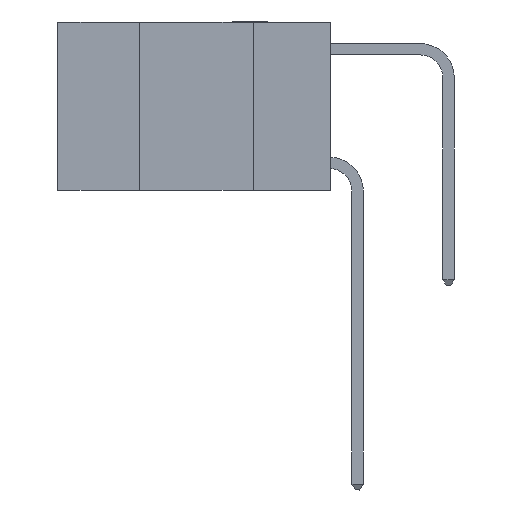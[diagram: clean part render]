
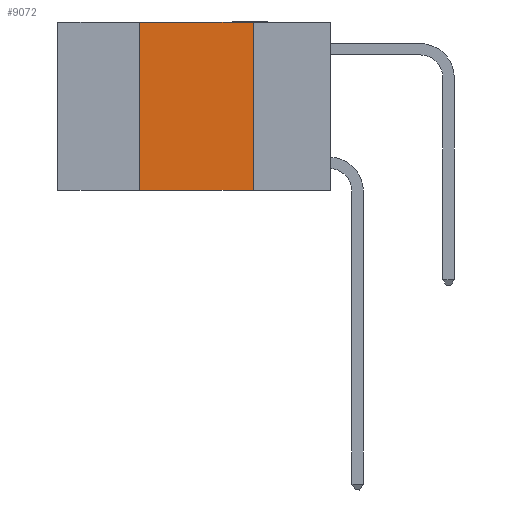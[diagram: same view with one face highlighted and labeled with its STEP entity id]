
A CAD part, left-side view. The second image highlights one B-rep face of the part: STEP entity #9072.
In plain terms, the highlighted planar face has unit normal (-1, 0, 0).
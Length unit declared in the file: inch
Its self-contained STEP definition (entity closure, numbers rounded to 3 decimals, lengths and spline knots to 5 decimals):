
#409 = CARTESIAN_POINT ( 'NONE',  ( 0., 0.42, 0. ) ) ;
#1998 = ORIENTED_EDGE ( 'NONE', *, *, #14082, .F. ) ;
#2023 = DIRECTION ( 'NONE',  ( 0., -1., 0. ) ) ;
#2148 = PLANE ( 'NONE',  #6805 ) ;
#3165 = ORIENTED_EDGE ( 'NONE', *, *, #5633, .F. ) ;
#3725 = LINE ( 'NONE', #13849, #8418 ) ;
#4829 = CARTESIAN_POINT ( 'NONE',  ( 0., 0.42, -0.37 ) ) ;
#5521 = VERTEX_POINT ( 'NONE', #15362 ) ;
#5633 = EDGE_CURVE ( 'NONE', #11752, #13836, #15517, .T. ) ;
#5691 = EDGE_LOOP ( 'NONE', ( #15381, #1998, #3165, #9033 ) ) ;
#5733 = EDGE_CURVE ( 'NONE', #11752, #10014, #7195, .T. ) ;
#5978 = DIRECTION ( 'NONE',  ( 0., 0., -1. ) ) ;
#6142 = DIRECTION ( 'NONE',  ( 0., 0., -1. ) ) ;
#6805 = AXIS2_PLACEMENT_3D ( 'NONE', #7239, #12229, #5978 ) ;
#7195 = LINE ( 'NONE', #13567, #16121 ) ;
#7239 = CARTESIAN_POINT ( 'NONE',  ( 0., 0.6, 0. ) ) ;
#8418 = VECTOR ( 'NONE', #6142, 39.37008 ) ;
#8916 = LINE ( 'NONE', #13835, #11642 ) ;
#9033 = ORIENTED_EDGE ( 'NONE', *, *, #5733, .T. ) ;
#9072 = ADVANCED_FACE ( 'NONE', ( #10893 ), #2148, .F. ) ;
#9412 = CARTESIAN_POINT ( 'NONE',  ( 0., 0.42, 0. ) ) ;
#9589 = EDGE_CURVE ( 'NONE', #5521, #10014, #3725, .T. ) ;
#10014 = VERTEX_POINT ( 'NONE', #16158 ) ;
#10372 = DIRECTION ( 'NONE',  ( 0., 0., 1. ) ) ;
#10893 = FACE_OUTER_BOUND ( 'NONE', #5691, .T. ) ;
#11642 = VECTOR ( 'NONE', #12528, 39.37008 ) ;
#11752 = VERTEX_POINT ( 'NONE', #4829 ) ;
#12229 = DIRECTION ( 'NONE',  ( 1., 0., 0. ) ) ;
#12421 = VECTOR ( 'NONE', #10372, 39.37008 ) ;
#12528 = DIRECTION ( 'NONE',  ( 0., -1., 0. ) ) ;
#13567 = CARTESIAN_POINT ( 'NONE',  ( 0., 0.6, -0.37 ) ) ;
#13836 = VERTEX_POINT ( 'NONE', #409 ) ;
#13835 = CARTESIAN_POINT ( 'NONE',  ( 0., 0.6, 0. ) ) ;
#13849 = CARTESIAN_POINT ( 'NONE',  ( 0., 0.17, 0. ) ) ;
#14082 = EDGE_CURVE ( 'NONE', #13836, #5521, #8916, .T. ) ;
#15362 = CARTESIAN_POINT ( 'NONE',  ( 0., 0.17, 0. ) ) ;
#15381 = ORIENTED_EDGE ( 'NONE', *, *, #9589, .F. ) ;
#15517 = LINE ( 'NONE', #9412, #12421 ) ;
#16121 = VECTOR ( 'NONE', #2023, 39.37008 ) ;
#16158 = CARTESIAN_POINT ( 'NONE',  ( 0., 0.17, -0.37 ) ) ;
